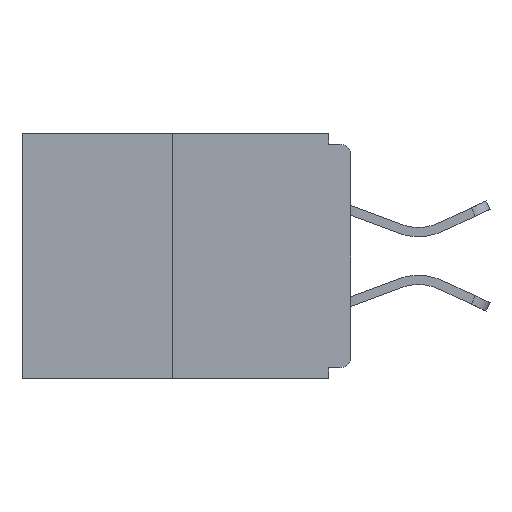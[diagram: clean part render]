
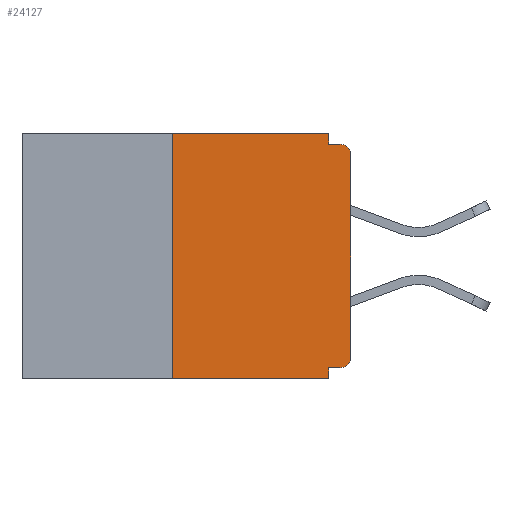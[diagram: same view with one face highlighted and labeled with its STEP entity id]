
A CAD part, left-side view. The second image highlights one B-rep face of the part: STEP entity #24127.
In plain terms, the highlighted planar face has unit normal (-1, 0, 0).
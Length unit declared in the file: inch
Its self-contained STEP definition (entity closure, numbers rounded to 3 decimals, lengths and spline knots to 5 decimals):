
#66 = VERTEX_POINT ( 'NONE', #3599 ) ;
#797 = DIRECTION ( 'NONE',  ( 0., -1., 0. ) ) ;
#1460 = ORIENTED_EDGE ( 'NONE', *, *, #13564, .F. ) ;
#1813 = CARTESIAN_POINT ( 'NONE',  ( 0., 0.015, -0.313 ) ) ;
#1967 = DIRECTION ( 'NONE',  ( -1., 0., 0. ) ) ;
#2324 = CARTESIAN_POINT ( 'NONE',  ( 0., 0.25, 0. ) ) ;
#2372 = LINE ( 'NONE', #18278, #9131 ) ;
#2742 = DIRECTION ( 'NONE',  ( 0., 0., -1. ) ) ;
#2897 = CIRCLE ( 'NONE', #12437, 0.015 ) ;
#3394 = EDGE_LOOP ( 'NONE', ( #16016, #8133, #4694, #5082, #18194, #12572, #9481, #22012, #1460, #11348 ) ) ;
#3599 = CARTESIAN_POINT ( 'NONE',  ( 0., 0., -0.03 ) ) ;
#3654 = EDGE_CURVE ( 'NONE', #21696, #66, #18966, .T. ) ;
#4694 = ORIENTED_EDGE ( 'NONE', *, *, #11076, .T. ) ;
#5082 = ORIENTED_EDGE ( 'NONE', *, *, #5604, .F. ) ;
#5326 = CARTESIAN_POINT ( 'NONE',  ( 0., 0.031, -0.015 ) ) ;
#5578 = DIRECTION ( 'NONE',  ( 0., 0., 1. ) ) ;
#5604 = EDGE_CURVE ( 'NONE', #8299, #18148, #13358, .T. ) ;
#6708 = EDGE_CURVE ( 'NONE', #10403, #21317, #14599, .T. ) ;
#7060 = LINE ( 'NONE', #13101, #13186 ) ;
#7363 = CARTESIAN_POINT ( 'NONE',  ( 0., 0.25, 0. ) ) ;
#7521 = VECTOR ( 'NONE', #5578, 39.37008 ) ;
#7960 = CARTESIAN_POINT ( 'NONE',  ( 0., 0., -0.015 ) ) ;
#8036 = EDGE_CURVE ( 'NONE', #12848, #21696, #2897, .T. ) ;
#8052 = DIRECTION ( 'NONE',  ( 0., -1., 0. ) ) ;
#8133 = ORIENTED_EDGE ( 'NONE', *, *, #22836, .F. ) ;
#8299 = VERTEX_POINT ( 'NONE', #14671 ) ;
#9131 = VECTOR ( 'NONE', #26618, 39.37008 ) ;
#9481 = ORIENTED_EDGE ( 'NONE', *, *, #3654, .T. ) ;
#10403 = VERTEX_POINT ( 'NONE', #21995 ) ;
#10961 = EDGE_CURVE ( 'NONE', #66, #25630, #15792, .T. ) ;
#11076 = EDGE_CURVE ( 'NONE', #25760, #18148, #7060, .T. ) ;
#11348 = ORIENTED_EDGE ( 'NONE', *, *, #6708, .F. ) ;
#11529 = DIRECTION ( 'NONE',  ( 0., 0., -1. ) ) ;
#11952 = DIRECTION ( 'NONE',  ( -1., 0., 0. ) ) ;
#12195 = CARTESIAN_POINT ( 'NONE',  ( 0., 0.015, -0.328 ) ) ;
#12437 = AXIS2_PLACEMENT_3D ( 'NONE', #1813, #11952, #2742 ) ;
#12572 = ORIENTED_EDGE ( 'NONE', *, *, #8036, .T. ) ;
#12848 = VERTEX_POINT ( 'NONE', #12195 ) ;
#13011 = LINE ( 'NONE', #7363, #7521 ) ;
#13101 = CARTESIAN_POINT ( 'NONE',  ( 0., 0.46, -0.343 ) ) ;
#13186 = VECTOR ( 'NONE', #797, 39.37008 ) ;
#13358 = LINE ( 'NONE', #26493, #16605 ) ;
#13564 = EDGE_CURVE ( 'NONE', #21317, #25630, #18188, .T. ) ;
#13942 = VECTOR ( 'NONE', #11529, 39.37008 ) ;
#14279 = CARTESIAN_POINT ( 'NONE',  ( 0., 0.015, -0.03 ) ) ;
#14398 = CARTESIAN_POINT ( 'NONE',  ( 0., 0., 0. ) ) ;
#14599 = LINE ( 'NONE', #21831, #13942 ) ;
#14671 = CARTESIAN_POINT ( 'NONE',  ( 0., 0.031, -0.328 ) ) ;
#15792 = CIRCLE ( 'NONE', #17967, 0.015 ) ;
#16016 = ORIENTED_EDGE ( 'NONE', *, *, #25249, .F. ) ;
#16023 = CARTESIAN_POINT ( 'NONE',  ( 0., 0.46, 0. ) ) ;
#16362 = DIRECTION ( 'NONE',  ( 0., 0., -1. ) ) ;
#16605 = VECTOR ( 'NONE', #24232, 39.37008 ) ;
#16946 = DIRECTION ( 'NONE',  ( 0., -1., 0. ) ) ;
#17967 = AXIS2_PLACEMENT_3D ( 'NONE', #14279, #1967, #16362 ) ;
#18148 = VERTEX_POINT ( 'NONE', #18377 ) ;
#18158 = DIRECTION ( 'NONE',  ( 1., 0., 0. ) ) ;
#18188 = LINE ( 'NONE', #7960, #22430 ) ;
#18194 = ORIENTED_EDGE ( 'NONE', *, *, #22950, .F. ) ;
#18254 = DIRECTION ( 'NONE',  ( 0., 0., -1. ) ) ;
#18262 = DIRECTION ( 'NONE',  ( 0., 0., 1. ) ) ;
#18278 = CARTESIAN_POINT ( 'NONE',  ( 0., 0., -0.328 ) ) ;
#18377 = CARTESIAN_POINT ( 'NONE',  ( 0., 0.031, -0.343 ) ) ;
#18665 = VECTOR ( 'NONE', #16946, 39.37008 ) ;
#18966 = LINE ( 'NONE', #14398, #19622 ) ;
#18991 = CARTESIAN_POINT ( 'NONE',  ( 0., 0.015, -0.015 ) ) ;
#19299 = VERTEX_POINT ( 'NONE', #2324 ) ;
#19622 = VECTOR ( 'NONE', #18262, 39.37008 ) ;
#19636 = CARTESIAN_POINT ( 'NONE',  ( 0., 0., -0.313 ) ) ;
#20697 = FACE_OUTER_BOUND ( 'NONE', #3394, .T. ) ;
#21317 = VERTEX_POINT ( 'NONE', #5326 ) ;
#21696 = VERTEX_POINT ( 'NONE', #19636 ) ;
#21831 = CARTESIAN_POINT ( 'NONE',  ( 0., 0.031, 0. ) ) ;
#21995 = CARTESIAN_POINT ( 'NONE',  ( 0., 0.031, 0. ) ) ;
#22012 = ORIENTED_EDGE ( 'NONE', *, *, #10961, .T. ) ;
#22430 = VECTOR ( 'NONE', #8052, 39.37008 ) ;
#22509 = AXIS2_PLACEMENT_3D ( 'NONE', #16023, #18158, #18254 ) ;
#22836 = EDGE_CURVE ( 'NONE', #25760, #19299, #13011, .T. ) ;
#22950 = EDGE_CURVE ( 'NONE', #12848, #8299, #2372, .T. ) ;
#24127 = ADVANCED_FACE ( 'NONE', ( #20697 ), #26401, .F. ) ;
#24177 = LINE ( 'NONE', #25171, #18665 ) ;
#24232 = DIRECTION ( 'NONE',  ( 0., 0., -1. ) ) ;
#25171 = CARTESIAN_POINT ( 'NONE',  ( 0., 0.46, 0. ) ) ;
#25249 = EDGE_CURVE ( 'NONE', #19299, #10403, #24177, .T. ) ;
#25497 = CARTESIAN_POINT ( 'NONE',  ( 0., 0.25, -0.343 ) ) ;
#25630 = VERTEX_POINT ( 'NONE', #18991 ) ;
#25760 = VERTEX_POINT ( 'NONE', #25497 ) ;
#26401 = PLANE ( 'NONE',  #22509 ) ;
#26493 = CARTESIAN_POINT ( 'NONE',  ( 0., 0.031, -0.343 ) ) ;
#26618 = DIRECTION ( 'NONE',  ( 0., 1., 0. ) ) ;
